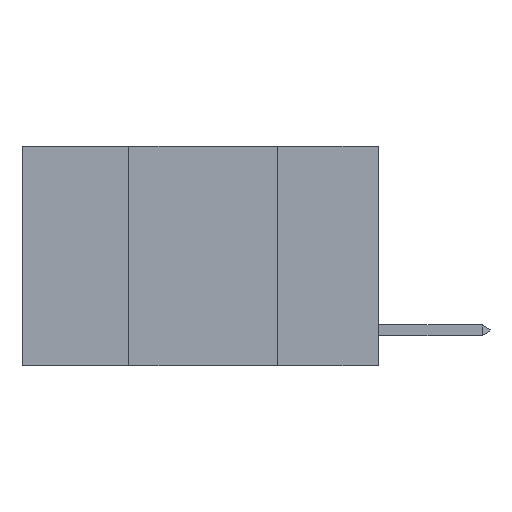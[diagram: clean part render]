
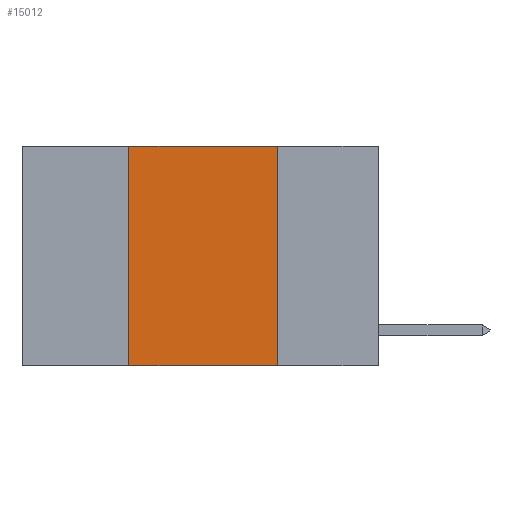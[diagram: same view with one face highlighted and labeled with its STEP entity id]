
A CAD part, left-side view. The second image highlights one B-rep face of the part: STEP entity #15012.
In plain terms, the highlighted planar face has unit normal (-1, 0, 0).
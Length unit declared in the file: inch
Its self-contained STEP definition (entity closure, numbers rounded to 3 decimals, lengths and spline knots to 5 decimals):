
#95 = ORIENTED_EDGE ( 'NONE', *, *, #19873, .F. ) ;
#2712 = LINE ( 'NONE', #12694, #7231 ) ;
#3327 = CARTESIAN_POINT ( 'NONE',  ( 0., 0.6, 0. ) ) ;
#5228 = DIRECTION ( 'NONE',  ( 0., 0., -1. ) ) ;
#5232 = ORIENTED_EDGE ( 'NONE', *, *, #10804, .T. ) ;
#6853 = DIRECTION ( 'NONE',  ( 0., -1., 0. ) ) ;
#7231 = VECTOR ( 'NONE', #12773, 39.37008 ) ;
#7300 = LINE ( 'NONE', #15556, #22065 ) ;
#7402 = CARTESIAN_POINT ( 'NONE',  ( 0., 0.42, 0. ) ) ;
#7754 = DIRECTION ( 'NONE',  ( 0., -1., 0. ) ) ;
#8137 = LINE ( 'NONE', #11690, #12751 ) ;
#8953 = VERTEX_POINT ( 'NONE', #13481 ) ;
#10364 = LINE ( 'NONE', #20434, #17320 ) ;
#10804 = EDGE_CURVE ( 'NONE', #17668, #13562, #10364, .T. ) ;
#11690 = CARTESIAN_POINT ( 'NONE',  ( 0., 0.17, 0. ) ) ;
#11782 = DIRECTION ( 'NONE',  ( 0., 0., -1. ) ) ;
#12694 = CARTESIAN_POINT ( 'NONE',  ( 0., 0.42, 0. ) ) ;
#12751 = VECTOR ( 'NONE', #11782, 39.37008 ) ;
#12773 = DIRECTION ( 'NONE',  ( 0., 0., 1. ) ) ;
#13481 = CARTESIAN_POINT ( 'NONE',  ( 0., 0.17, 0. ) ) ;
#13562 = VERTEX_POINT ( 'NONE', #23463 ) ;
#15012 = ADVANCED_FACE ( 'NONE', ( #20762 ), #15023, .F. ) ;
#15023 = PLANE ( 'NONE',  #24031 ) ;
#15556 = CARTESIAN_POINT ( 'NONE',  ( 0., 0.6, 0. ) ) ;
#16967 = DIRECTION ( 'NONE',  ( 1., 0., 0. ) ) ;
#17320 = VECTOR ( 'NONE', #6853, 39.37008 ) ;
#17668 = VERTEX_POINT ( 'NONE', #18164 ) ;
#17804 = ORIENTED_EDGE ( 'NONE', *, *, #24165, .F. ) ;
#18164 = CARTESIAN_POINT ( 'NONE',  ( 0., 0.42, -0.37 ) ) ;
#19873 = EDGE_CURVE ( 'NONE', #17668, #20126, #2712, .T. ) ;
#20126 = VERTEX_POINT ( 'NONE', #7402 ) ;
#20434 = CARTESIAN_POINT ( 'NONE',  ( 0., 0.6, -0.37 ) ) ;
#20762 = FACE_OUTER_BOUND ( 'NONE', #22829, .T. ) ;
#21101 = EDGE_CURVE ( 'NONE', #8953, #13562, #8137, .T. ) ;
#22065 = VECTOR ( 'NONE', #7754, 39.37008 ) ;
#22829 = EDGE_LOOP ( 'NONE', ( #24123, #17804, #95, #5232 ) ) ;
#23463 = CARTESIAN_POINT ( 'NONE',  ( 0., 0.17, -0.37 ) ) ;
#24031 = AXIS2_PLACEMENT_3D ( 'NONE', #3327, #16967, #5228 ) ;
#24123 = ORIENTED_EDGE ( 'NONE', *, *, #21101, .F. ) ;
#24165 = EDGE_CURVE ( 'NONE', #20126, #8953, #7300, .T. ) ;
